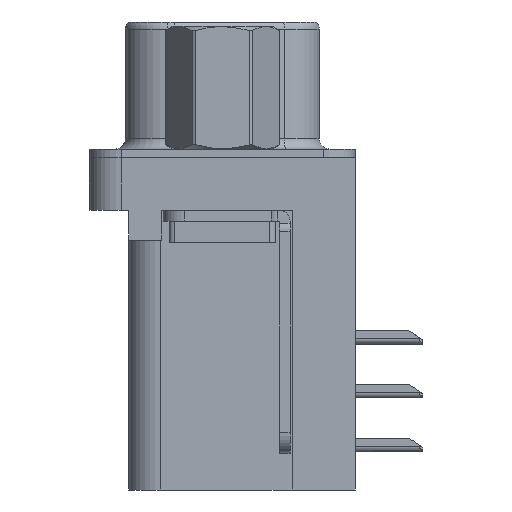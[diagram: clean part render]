
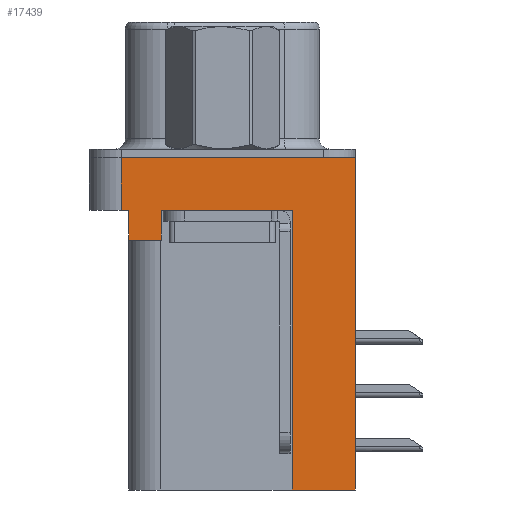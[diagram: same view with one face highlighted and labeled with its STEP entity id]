
A CAD part, left-side view. The second image highlights one B-rep face of the part: STEP entity #17439.
In plain terms, the highlighted planar face has unit normal (-1, 0, 0).
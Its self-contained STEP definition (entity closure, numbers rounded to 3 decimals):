
#846 = EDGE_CURVE ( 'NONE', #7145, #10646, #19314, .T. ) ;
#907 = VERTEX_POINT ( 'NONE', #26121 ) ;
#2037 = VECTOR ( 'NONE', #27482, 1000. ) ;
#2433 = ORIENTED_EDGE ( 'NONE', *, *, #18660, .F. ) ;
#2868 = ORIENTED_EDGE ( 'NONE', *, *, #14713, .T. ) ;
#2942 = DIRECTION ( 'NONE',  ( 0., 0., 1. ) ) ;
#3368 = EDGE_CURVE ( 'NONE', #14556, #15047, #8499, .T. ) ;
#3749 = EDGE_CURVE ( 'NONE', #10646, #21114, #22650, .T. ) ;
#4952 = CARTESIAN_POINT ( 'NONE',  ( -2.935, 2.895, -3.9 ) ) ;
#5139 = CARTESIAN_POINT ( 'NONE',  ( -2.935, -3.295, -15.7 ) ) ;
#5355 = ORIENTED_EDGE ( 'NONE', *, *, #3368, .F. ) ;
#5702 = CARTESIAN_POINT ( 'NONE',  ( -2.935, 4.775, -2.5 ) ) ;
#5801 = DIRECTION ( 'NONE',  ( 0., 0., 1. ) ) ;
#5857 = DIRECTION ( 'NONE',  ( 0., 0., 1. ) ) ;
#7109 = ORIENTED_EDGE ( 'NONE', *, *, #8665, .F. ) ;
#7114 = VECTOR ( 'NONE', #5801, 1000. ) ;
#7145 = VERTEX_POINT ( 'NONE', #15509 ) ;
#7535 = LINE ( 'NONE', #23570, #24096 ) ;
#7882 = CARTESIAN_POINT ( 'NONE',  ( -2.935, -6.275, -2.5 ) ) ;
#8469 = DIRECTION ( 'NONE',  ( 0., 0., 1. ) ) ;
#8499 = LINE ( 'NONE', #20398, #2037 ) ;
#8665 = EDGE_CURVE ( 'NONE', #15047, #23671, #9305, .T. ) ;
#8726 = DIRECTION ( 'NONE',  ( 0., 0., 1. ) ) ;
#9031 = CARTESIAN_POINT ( 'NONE',  ( -2.935, 4.425, -3.9 ) ) ;
#9305 = LINE ( 'NONE', #15979, #26919 ) ;
#10237 = LINE ( 'NONE', #9031, #21063 ) ;
#10399 = CARTESIAN_POINT ( 'NONE',  ( -2.935, -6.275, -2.5 ) ) ;
#10646 = VERTEX_POINT ( 'NONE', #23254 ) ;
#10869 = ORIENTED_EDGE ( 'NONE', *, *, #25708, .T. ) ;
#11054 = EDGE_LOOP ( 'NONE', ( #13233, #19257, #12264, #15735, #2433, #2868, #16482, #7109, #5355, #10869 ) ) ;
#11218 = DIRECTION ( 'NONE',  ( 0., -1., 0. ) ) ;
#11567 = VERTEX_POINT ( 'NONE', #15655 ) ;
#11585 = CARTESIAN_POINT ( 'NONE',  ( -2.935, -3.295, -2.5 ) ) ;
#11661 = DIRECTION ( 'NONE',  ( 0., -1., 0. ) ) ;
#12264 = ORIENTED_EDGE ( 'NONE', *, *, #17759, .T. ) ;
#12566 = LINE ( 'NONE', #26372, #18299 ) ;
#12608 = DIRECTION ( 'NONE',  ( -1., 0., 0. ) ) ;
#13233 = ORIENTED_EDGE ( 'NONE', *, *, #3749, .F. ) ;
#13238 = CARTESIAN_POINT ( 'NONE',  ( -2.935, -6.275, 0. ) ) ;
#13369 = VECTOR ( 'NONE', #8726, 1000. ) ;
#14314 = CARTESIAN_POINT ( 'NONE',  ( -2.935, -6.275, 0. ) ) ;
#14556 = VERTEX_POINT ( 'NONE', #18799 ) ;
#14713 = EDGE_CURVE ( 'NONE', #18758, #907, #7535, .T. ) ;
#15047 = VERTEX_POINT ( 'NONE', #5139 ) ;
#15096 = EDGE_CURVE ( 'NONE', #907, #23671, #16708, .T. ) ;
#15385 = CARTESIAN_POINT ( 'NONE',  ( -2.935, -6.275, -2.5 ) ) ;
#15509 = CARTESIAN_POINT ( 'NONE',  ( -2.935, 4.775, -2.5 ) ) ;
#15644 = LINE ( 'NONE', #20983, #20663 ) ;
#15655 = CARTESIAN_POINT ( 'NONE',  ( -2.935, 4.425, -3.9 ) ) ;
#15735 = ORIENTED_EDGE ( 'NONE', *, *, #17385, .F. ) ;
#15979 = CARTESIAN_POINT ( 'NONE',  ( -2.935, -3.295, -15.7 ) ) ;
#16482 = ORIENTED_EDGE ( 'NONE', *, *, #15096, .T. ) ;
#16708 = LINE ( 'NONE', #7882, #22384 ) ;
#17385 = EDGE_CURVE ( 'NONE', #11567, #27141, #15644, .T. ) ;
#17439 = ADVANCED_FACE ( 'NONE', ( #25049 ), #23303, .T. ) ;
#17645 = VECTOR ( 'NONE', #11661, 1000. ) ;
#17759 = EDGE_CURVE ( 'NONE', #7145, #27141, #12566, .T. ) ;
#18299 = VECTOR ( 'NONE', #11218, 1000. ) ;
#18660 = EDGE_CURVE ( 'NONE', #18758, #11567, #10237, .T. ) ;
#18758 = VERTEX_POINT ( 'NONE', #4952 ) ;
#18799 = CARTESIAN_POINT ( 'NONE',  ( -2.935, -6.275, -15.7 ) ) ;
#19257 = ORIENTED_EDGE ( 'NONE', *, *, #846, .F. ) ;
#19314 = LINE ( 'NONE', #5702, #7114 ) ;
#19814 = DIRECTION ( 'NONE',  ( 0., 1., 0. ) ) ;
#20398 = CARTESIAN_POINT ( 'NONE',  ( -2.935, -3.295, -15.7 ) ) ;
#20663 = VECTOR ( 'NONE', #5857, 1000. ) ;
#20983 = CARTESIAN_POINT ( 'NONE',  ( -2.935, 4.425, -3.9 ) ) ;
#21063 = VECTOR ( 'NONE', #19814, 1000. ) ;
#21114 = VERTEX_POINT ( 'NONE', #14314 ) ;
#22384 = VECTOR ( 'NONE', #22986, 1000. ) ;
#22650 = LINE ( 'NONE', #13238, #17645 ) ;
#22986 = DIRECTION ( 'NONE',  ( 0., -1., 0. ) ) ;
#23253 = AXIS2_PLACEMENT_3D ( 'NONE', #10399, #12608, #27759 ) ;
#23254 = CARTESIAN_POINT ( 'NONE',  ( -2.935, 4.775, 0. ) ) ;
#23303 = PLANE ( 'NONE',  #23253 ) ;
#23570 = CARTESIAN_POINT ( 'NONE',  ( -2.935, 2.895, -3.9 ) ) ;
#23671 = VERTEX_POINT ( 'NONE', #11585 ) ;
#24096 = VECTOR ( 'NONE', #8469, 1000. ) ;
#24313 = CARTESIAN_POINT ( 'NONE',  ( -2.935, 4.425, -2.5 ) ) ;
#24828 = LINE ( 'NONE', #15385, #13369 ) ;
#25049 = FACE_OUTER_BOUND ( 'NONE', #11054, .T. ) ;
#25708 = EDGE_CURVE ( 'NONE', #14556, #21114, #24828, .T. ) ;
#26121 = CARTESIAN_POINT ( 'NONE',  ( -2.935, 2.895, -2.5 ) ) ;
#26372 = CARTESIAN_POINT ( 'NONE',  ( -2.935, -6.275, -2.5 ) ) ;
#26919 = VECTOR ( 'NONE', #2942, 1000. ) ;
#27141 = VERTEX_POINT ( 'NONE', #24313 ) ;
#27482 = DIRECTION ( 'NONE',  ( 0., 1., 0. ) ) ;
#27759 = DIRECTION ( 'NONE',  ( 0., 0., 1. ) ) ;
